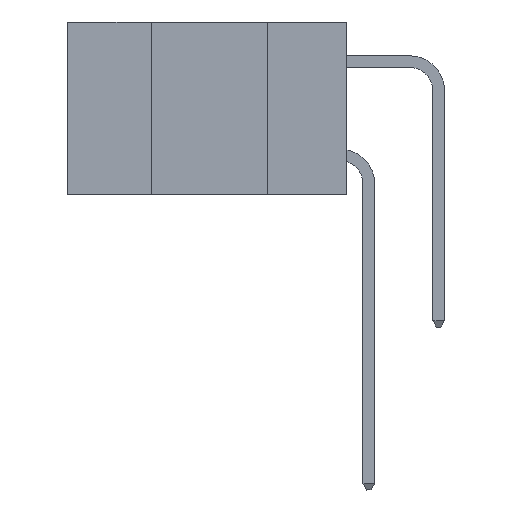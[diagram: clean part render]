
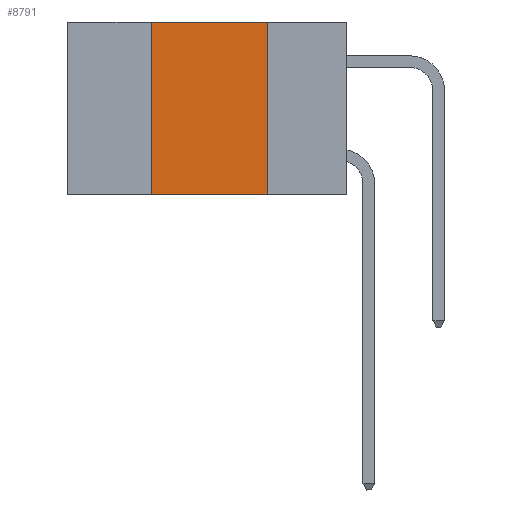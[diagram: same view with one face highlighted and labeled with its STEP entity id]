
A CAD part, left-side view. The second image highlights one B-rep face of the part: STEP entity #8791.
In plain terms, the highlighted planar face has unit normal (-1, 0, 0).
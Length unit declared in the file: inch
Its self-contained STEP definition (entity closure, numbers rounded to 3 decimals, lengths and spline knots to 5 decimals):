
#101 = VERTEX_POINT ( 'NONE', #2562 ) ;
#639 = EDGE_CURVE ( 'NONE', #13348, #16393, #15739, .T. ) ;
#1077 = CARTESIAN_POINT ( 'NONE',  ( 0., 0.17, 0. ) ) ;
#2053 = LINE ( 'NONE', #9334, #9257 ) ;
#2256 = VERTEX_POINT ( 'NONE', #1077 ) ;
#2562 = CARTESIAN_POINT ( 'NONE',  ( 0., 0.17, -0.37 ) ) ;
#3202 = CARTESIAN_POINT ( 'NONE',  ( 0., 0.6, 0. ) ) ;
#4058 = DIRECTION ( 'NONE',  ( 0., -1., 0. ) ) ;
#4606 = LINE ( 'NONE', #8750, #8744 ) ;
#5799 = VECTOR ( 'NONE', #13538, 39.37008 ) ;
#6304 = PLANE ( 'NONE',  #10382 ) ;
#6412 = DIRECTION ( 'NONE',  ( 1., 0., 0. ) ) ;
#6969 = EDGE_LOOP ( 'NONE', ( #20538, #13356, #8661, #14607 ) ) ;
#8661 = ORIENTED_EDGE ( 'NONE', *, *, #639, .F. ) ;
#8744 = VECTOR ( 'NONE', #23368, 39.37008 ) ;
#8750 = CARTESIAN_POINT ( 'NONE',  ( 0., 0.17, 0. ) ) ;
#8791 = ADVANCED_FACE ( 'NONE', ( #19496 ), #6304, .F. ) ;
#9243 = EDGE_CURVE ( 'NONE', #16393, #2256, #22803, .T. ) ;
#9257 = VECTOR ( 'NONE', #4058, 39.37008 ) ;
#9334 = CARTESIAN_POINT ( 'NONE',  ( 0., 0.6, -0.37 ) ) ;
#10382 = AXIS2_PLACEMENT_3D ( 'NONE', #3202, #6412, #12122 ) ;
#12122 = DIRECTION ( 'NONE',  ( 0., 0., -1. ) ) ;
#12306 = CARTESIAN_POINT ( 'NONE',  ( 0., 0.42, 0. ) ) ;
#12980 = EDGE_CURVE ( 'NONE', #2256, #101, #4606, .T. ) ;
#13262 = CARTESIAN_POINT ( 'NONE',  ( 0., 0.42, 0. ) ) ;
#13348 = VERTEX_POINT ( 'NONE', #13947 ) ;
#13356 = ORIENTED_EDGE ( 'NONE', *, *, #9243, .F. ) ;
#13538 = DIRECTION ( 'NONE',  ( 0., -1., 0. ) ) ;
#13658 = CARTESIAN_POINT ( 'NONE',  ( 0., 0.6, 0. ) ) ;
#13947 = CARTESIAN_POINT ( 'NONE',  ( 0., 0.42, -0.37 ) ) ;
#14607 = ORIENTED_EDGE ( 'NONE', *, *, #22307, .T. ) ;
#15739 = LINE ( 'NONE', #12306, #16272 ) ;
#16272 = VECTOR ( 'NONE', #23355, 39.37008 ) ;
#16393 = VERTEX_POINT ( 'NONE', #13262 ) ;
#19496 = FACE_OUTER_BOUND ( 'NONE', #6969, .T. ) ;
#20538 = ORIENTED_EDGE ( 'NONE', *, *, #12980, .F. ) ;
#22307 = EDGE_CURVE ( 'NONE', #13348, #101, #2053, .T. ) ;
#22803 = LINE ( 'NONE', #13658, #5799 ) ;
#23355 = DIRECTION ( 'NONE',  ( 0., 0., 1. ) ) ;
#23368 = DIRECTION ( 'NONE',  ( 0., 0., -1. ) ) ;
